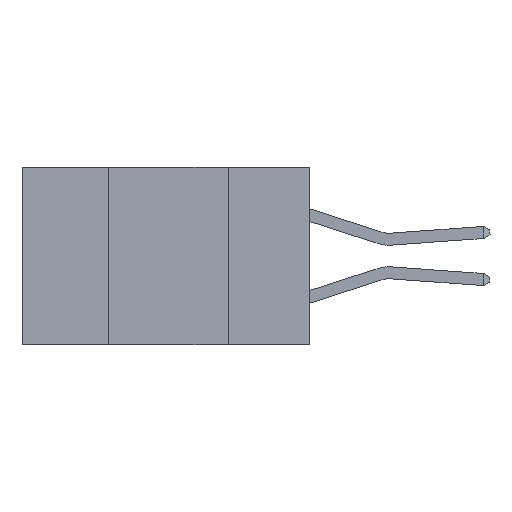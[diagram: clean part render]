
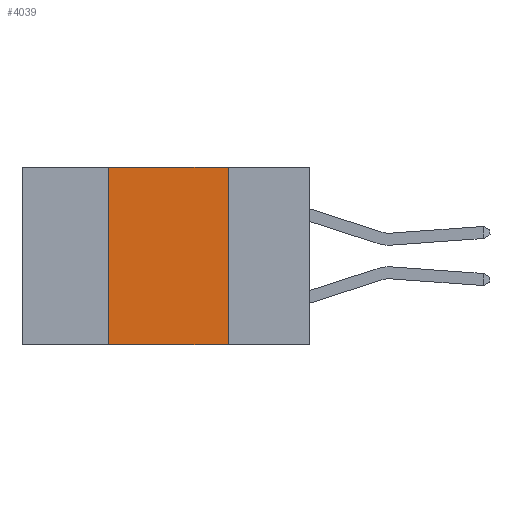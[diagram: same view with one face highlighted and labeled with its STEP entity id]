
A CAD part, left-side view. The second image highlights one B-rep face of the part: STEP entity #4039.
In plain terms, the highlighted planar face has unit normal (-1, 0, 0).
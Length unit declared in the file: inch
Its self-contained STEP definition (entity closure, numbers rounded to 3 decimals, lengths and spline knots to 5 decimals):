
#292 = PLANE ( 'NONE',  #6714 ) ;
#350 = VECTOR ( 'NONE', #3143, 39.37008 ) ;
#806 = CARTESIAN_POINT ( 'NONE',  ( 0., 0.42, -0.37 ) ) ;
#1166 = EDGE_CURVE ( 'NONE', #1410, #3620, #1914, .T. ) ;
#1410 = VERTEX_POINT ( 'NONE', #10384 ) ;
#1880 = EDGE_LOOP ( 'NONE', ( #11989, #6298, #7629, #5794 ) ) ;
#1914 = LINE ( 'NONE', #6233, #7452 ) ;
#2239 = VERTEX_POINT ( 'NONE', #12460 ) ;
#2643 = EDGE_CURVE ( 'NONE', #6346, #2239, #7903, .T. ) ;
#2967 = LINE ( 'NONE', #8577, #350 ) ;
#3143 = DIRECTION ( 'NONE',  ( 0., -1., 0. ) ) ;
#3215 = DIRECTION ( 'NONE',  ( 0., 0., -1. ) ) ;
#3620 = VERTEX_POINT ( 'NONE', #7144 ) ;
#4039 = ADVANCED_FACE ( 'NONE', ( #5337 ), #292, .F. ) ;
#5337 = FACE_OUTER_BOUND ( 'NONE', #1880, .T. ) ;
#5794 = ORIENTED_EDGE ( 'NONE', *, *, #6394, .T. ) ;
#6233 = CARTESIAN_POINT ( 'NONE',  ( 0., 0.17, 0. ) ) ;
#6298 = ORIENTED_EDGE ( 'NONE', *, *, #12553, .F. ) ;
#6346 = VERTEX_POINT ( 'NONE', #806 ) ;
#6394 = EDGE_CURVE ( 'NONE', #6346, #3620, #2967, .T. ) ;
#6714 = AXIS2_PLACEMENT_3D ( 'NONE', #13122, #13769, #13745 ) ;
#7144 = CARTESIAN_POINT ( 'NONE',  ( 0., 0.17, -0.37 ) ) ;
#7452 = VECTOR ( 'NONE', #3215, 39.37008 ) ;
#7629 = ORIENTED_EDGE ( 'NONE', *, *, #2643, .F. ) ;
#7903 = LINE ( 'NONE', #11001, #10698 ) ;
#8577 = CARTESIAN_POINT ( 'NONE',  ( 0., 0.6, -0.37 ) ) ;
#9442 = CARTESIAN_POINT ( 'NONE',  ( 0., 0.6, 0. ) ) ;
#10384 = CARTESIAN_POINT ( 'NONE',  ( 0., 0.17, 0. ) ) ;
#10491 = DIRECTION ( 'NONE',  ( 0., 0., 1. ) ) ;
#10698 = VECTOR ( 'NONE', #10491, 39.37008 ) ;
#11001 = CARTESIAN_POINT ( 'NONE',  ( 0., 0.42, 0. ) ) ;
#11197 = LINE ( 'NONE', #9442, #13294 ) ;
#11989 = ORIENTED_EDGE ( 'NONE', *, *, #1166, .F. ) ;
#12460 = CARTESIAN_POINT ( 'NONE',  ( 0., 0.42, 0. ) ) ;
#12553 = EDGE_CURVE ( 'NONE', #2239, #1410, #11197, .T. ) ;
#13122 = CARTESIAN_POINT ( 'NONE',  ( 0., 0.6, 0. ) ) ;
#13294 = VECTOR ( 'NONE', #13601, 39.37008 ) ;
#13601 = DIRECTION ( 'NONE',  ( 0., -1., 0. ) ) ;
#13745 = DIRECTION ( 'NONE',  ( 0., 0., -1. ) ) ;
#13769 = DIRECTION ( 'NONE',  ( 1., 0., 0. ) ) ;
